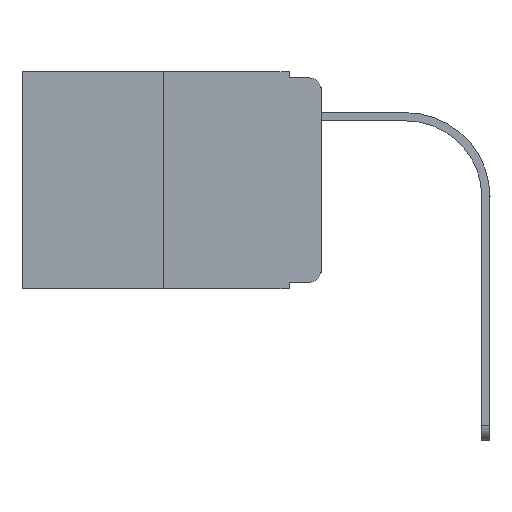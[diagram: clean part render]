
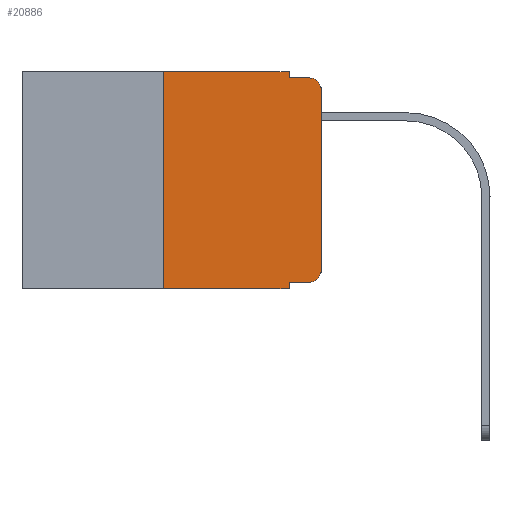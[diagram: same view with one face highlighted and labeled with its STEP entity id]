
A CAD part, left-side view. The second image highlights one B-rep face of the part: STEP entity #20886.
In plain terms, the highlighted planar face has unit normal (-1, 0, 0).
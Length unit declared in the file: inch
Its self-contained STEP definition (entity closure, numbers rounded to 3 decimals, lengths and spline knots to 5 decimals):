
#2 = DIRECTION ( 'NONE',  ( 0., 0., 1. ) ) ;
#522 = CARTESIAN_POINT ( 'NONE',  ( 0., 0.02, -0.03 ) ) ;
#648 = EDGE_CURVE ( 'NONE', #2170, #17892, #7872, .T. ) ;
#759 = FACE_OUTER_BOUND ( 'NONE', #9999, .T. ) ;
#882 = EDGE_CURVE ( 'NONE', #12157, #2833, #3220, .T. ) ;
#1081 = EDGE_CURVE ( 'NONE', #14709, #11397, #7920, .T. ) ;
#1100 = VECTOR ( 'NONE', #4426, 39.37008 ) ;
#1139 = ORIENTED_EDGE ( 'NONE', *, *, #11679, .T. ) ;
#1307 = CARTESIAN_POINT ( 'NONE',  ( 0., 0.051, -0.333 ) ) ;
#1373 = ORIENTED_EDGE ( 'NONE', *, *, #882, .T. ) ;
#1416 = AXIS2_PLACEMENT_3D ( 'NONE', #19349, #16026, #19245 ) ;
#1764 = VECTOR ( 'NONE', #11446, 39.37008 ) ;
#1816 = CIRCLE ( 'NONE', #16299, 0.02 ) ;
#2170 = VERTEX_POINT ( 'NONE', #9557 ) ;
#2699 = DIRECTION ( 'NONE',  ( 0., -1., 0. ) ) ;
#2833 = VERTEX_POINT ( 'NONE', #13439 ) ;
#3048 = EDGE_CURVE ( 'NONE', #6356, #17892, #9097, .T. ) ;
#3079 = VECTOR ( 'NONE', #6162, 39.37008 ) ;
#3220 = LINE ( 'NONE', #21495, #18804 ) ;
#3255 = DIRECTION ( 'NONE',  ( 0., 0., -1. ) ) ;
#3970 = LINE ( 'NONE', #1307, #16955 ) ;
#4426 = DIRECTION ( 'NONE',  ( 0., 0., -1. ) ) ;
#6086 = PLANE ( 'NONE',  #1416 ) ;
#6148 = CARTESIAN_POINT ( 'NONE',  ( 0., 0., -0.313 ) ) ;
#6162 = DIRECTION ( 'NONE',  ( 0., -1., 0. ) ) ;
#6356 = VERTEX_POINT ( 'NONE', #13936 ) ;
#6517 = CARTESIAN_POINT ( 'NONE',  ( 0., 0.051, -0.01 ) ) ;
#6723 = CARTESIAN_POINT ( 'NONE',  ( 0., 0.25, 0. ) ) ;
#6962 = ORIENTED_EDGE ( 'NONE', *, *, #9300, .F. ) ;
#7872 = LINE ( 'NONE', #9533, #1100 ) ;
#7920 = LINE ( 'NONE', #16546, #3079 ) ;
#8176 = DIRECTION ( 'NONE',  ( 0., 0., 1. ) ) ;
#8322 = ORIENTED_EDGE ( 'NONE', *, *, #1081, .F. ) ;
#8597 = ORIENTED_EDGE ( 'NONE', *, *, #3048, .T. ) ;
#9025 = CIRCLE ( 'NONE', #14682, 0.02 ) ;
#9097 = LINE ( 'NONE', #20963, #12267 ) ;
#9239 = EDGE_CURVE ( 'NONE', #2170, #14316, #3970, .T. ) ;
#9300 = EDGE_CURVE ( 'NONE', #6356, #14709, #20129, .T. ) ;
#9533 = CARTESIAN_POINT ( 'NONE',  ( 0., 0.051, 0. ) ) ;
#9557 = CARTESIAN_POINT ( 'NONE',  ( 0., 0.051, -0.333 ) ) ;
#9652 = CARTESIAN_POINT ( 'NONE',  ( 0., 0.051, 0. ) ) ;
#9978 = EDGE_CURVE ( 'NONE', #14038, #17877, #11499, .T. ) ;
#9999 = EDGE_LOOP ( 'NONE', ( #1373, #1139, #18271, #18502, #8322, #6962, #8597, #13193, #15973, #11801 ) ) ;
#11346 = DIRECTION ( 'NONE',  ( -1., 0., 0. ) ) ;
#11395 = DIRECTION ( 'NONE',  ( 0., -1., 0. ) ) ;
#11397 = VERTEX_POINT ( 'NONE', #9652 ) ;
#11403 = CARTESIAN_POINT ( 'NONE',  ( 0., 0.02, -0.01 ) ) ;
#11446 = DIRECTION ( 'NONE',  ( 0., 0., -1. ) ) ;
#11499 = LINE ( 'NONE', #6517, #20549 ) ;
#11606 = DIRECTION ( 'NONE',  ( 0., -1., 0. ) ) ;
#11679 = EDGE_CURVE ( 'NONE', #2833, #17877, #9025, .T. ) ;
#11801 = ORIENTED_EDGE ( 'NONE', *, *, #18793, .T. ) ;
#12157 = VERTEX_POINT ( 'NONE', #6148 ) ;
#12267 = VECTOR ( 'NONE', #2699, 39.37008 ) ;
#12708 = CARTESIAN_POINT ( 'NONE',  ( 0., 0.051, -0.343 ) ) ;
#12977 = LINE ( 'NONE', #19746, #1764 ) ;
#13193 = ORIENTED_EDGE ( 'NONE', *, *, #648, .F. ) ;
#13439 = CARTESIAN_POINT ( 'NONE',  ( 0., 0., -0.03 ) ) ;
#13936 = CARTESIAN_POINT ( 'NONE',  ( 0., 0.25, -0.343 ) ) ;
#14038 = VERTEX_POINT ( 'NONE', #14793 ) ;
#14294 = CARTESIAN_POINT ( 'NONE',  ( 0., 0.25, 0. ) ) ;
#14316 = VERTEX_POINT ( 'NONE', #16245 ) ;
#14682 = AXIS2_PLACEMENT_3D ( 'NONE', #522, #18785, #19001 ) ;
#14709 = VERTEX_POINT ( 'NONE', #14294 ) ;
#14793 = CARTESIAN_POINT ( 'NONE',  ( 0., 0.051, -0.01 ) ) ;
#15899 = VECTOR ( 'NONE', #8176, 39.37008 ) ;
#15973 = ORIENTED_EDGE ( 'NONE', *, *, #9239, .T. ) ;
#16026 = DIRECTION ( 'NONE',  ( 1., 0., 0. ) ) ;
#16245 = CARTESIAN_POINT ( 'NONE',  ( 0., 0.02, -0.333 ) ) ;
#16299 = AXIS2_PLACEMENT_3D ( 'NONE', #16423, #11346, #3255 ) ;
#16423 = CARTESIAN_POINT ( 'NONE',  ( 0., 0.02, -0.313 ) ) ;
#16546 = CARTESIAN_POINT ( 'NONE',  ( 0., 0.473, 0. ) ) ;
#16955 = VECTOR ( 'NONE', #11395, 39.37008 ) ;
#17877 = VERTEX_POINT ( 'NONE', #11403 ) ;
#17892 = VERTEX_POINT ( 'NONE', #12708 ) ;
#18271 = ORIENTED_EDGE ( 'NONE', *, *, #9978, .F. ) ;
#18502 = ORIENTED_EDGE ( 'NONE', *, *, #20150, .F. ) ;
#18785 = DIRECTION ( 'NONE',  ( -1., 0., 0. ) ) ;
#18793 = EDGE_CURVE ( 'NONE', #14316, #12157, #1816, .T. ) ;
#18804 = VECTOR ( 'NONE', #2, 39.37008 ) ;
#19001 = DIRECTION ( 'NONE',  ( 0., 0., -1. ) ) ;
#19245 = DIRECTION ( 'NONE',  ( 0., 0., -1. ) ) ;
#19349 = CARTESIAN_POINT ( 'NONE',  ( 0., 0.473, 0. ) ) ;
#19746 = CARTESIAN_POINT ( 'NONE',  ( 0., 0.051, 0. ) ) ;
#20129 = LINE ( 'NONE', #6723, #15899 ) ;
#20150 = EDGE_CURVE ( 'NONE', #11397, #14038, #12977, .T. ) ;
#20549 = VECTOR ( 'NONE', #11606, 39.37008 ) ;
#20886 = ADVANCED_FACE ( 'NONE', ( #759 ), #6086, .F. ) ;
#20963 = CARTESIAN_POINT ( 'NONE',  ( 0., 0.473, -0.343 ) ) ;
#21495 = CARTESIAN_POINT ( 'NONE',  ( 0., 0., 0. ) ) ;
